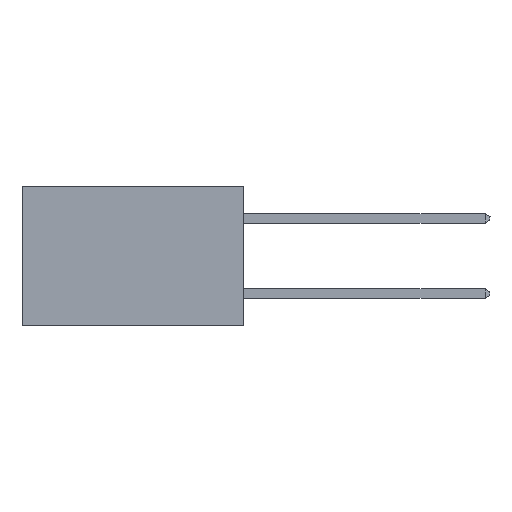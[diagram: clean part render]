
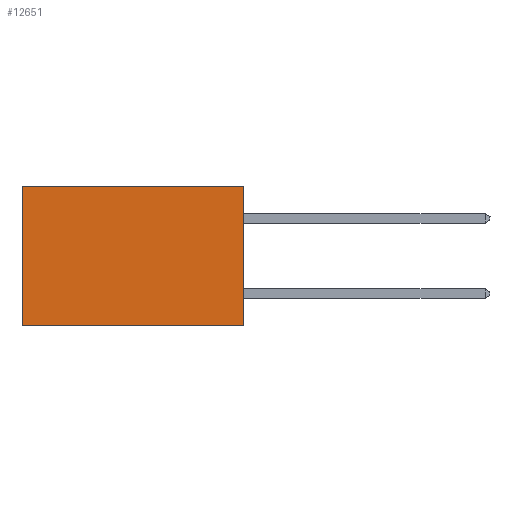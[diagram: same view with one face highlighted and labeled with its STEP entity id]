
A CAD part, left-side view. The second image highlights one B-rep face of the part: STEP entity #12651.
In plain terms, the highlighted planar face has unit normal (-1, 0, 0).
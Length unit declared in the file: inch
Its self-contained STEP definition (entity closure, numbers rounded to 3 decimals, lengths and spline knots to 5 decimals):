
#121 = VERTEX_POINT ( 'NONE', #4408 ) ;
#413 = LINE ( 'NONE', #1261, #7992 ) ;
#588 = CARTESIAN_POINT ( 'NONE',  ( 0.277, 0.59, -0.37 ) ) ;
#641 = CARTESIAN_POINT ( 'NONE',  ( 0.277, 0., -0.37 ) ) ;
#1136 = CARTESIAN_POINT ( 'NONE',  ( 0.277, 0., 0. ) ) ;
#1261 = CARTESIAN_POINT ( 'NONE',  ( 0.277, 0., -0.37 ) ) ;
#1402 = PLANE ( 'NONE',  #4136 ) ;
#2019 = VECTOR ( 'NONE', #10902, 39.37008 ) ;
#2558 = EDGE_CURVE ( 'NONE', #8640, #6250, #5430, .T. ) ;
#2584 = VERTEX_POINT ( 'NONE', #10808 ) ;
#3403 = ORIENTED_EDGE ( 'NONE', *, *, #12127, .T. ) ;
#3412 = DIRECTION ( 'NONE',  ( 1., 0., 0. ) ) ;
#4136 = AXIS2_PLACEMENT_3D ( 'NONE', #9654, #3412, #10673 ) ;
#4408 = CARTESIAN_POINT ( 'NONE',  ( 0.277, 0.59, 0. ) ) ;
#4541 = ORIENTED_EDGE ( 'NONE', *, *, #10246, .T. ) ;
#5396 = CARTESIAN_POINT ( 'NONE',  ( 0.277, 0., -0.37 ) ) ;
#5430 = LINE ( 'NONE', #5396, #8211 ) ;
#5576 = DIRECTION ( 'NONE',  ( 0., 1., 0. ) ) ;
#6250 = VERTEX_POINT ( 'NONE', #641 ) ;
#6359 = ORIENTED_EDGE ( 'NONE', *, *, #10726, .F. ) ;
#6680 = ORIENTED_EDGE ( 'NONE', *, *, #2558, .F. ) ;
#7402 = DIRECTION ( 'NONE',  ( 0., 1., 0. ) ) ;
#7992 = VECTOR ( 'NONE', #7402, 39.37008 ) ;
#8009 = LINE ( 'NONE', #9749, #10441 ) ;
#8211 = VECTOR ( 'NONE', #8912, 39.37008 ) ;
#8640 = VERTEX_POINT ( 'NONE', #1136 ) ;
#8912 = DIRECTION ( 'NONE',  ( 0., 0., -1. ) ) ;
#9593 = FACE_OUTER_BOUND ( 'NONE', #11273, .T. ) ;
#9654 = CARTESIAN_POINT ( 'NONE',  ( 0.277, 0., -0.37 ) ) ;
#9749 = CARTESIAN_POINT ( 'NONE',  ( 0.277, 0., 0. ) ) ;
#10246 = EDGE_CURVE ( 'NONE', #8640, #121, #8009, .T. ) ;
#10251 = LINE ( 'NONE', #588, #2019 ) ;
#10441 = VECTOR ( 'NONE', #5576, 39.37008 ) ;
#10673 = DIRECTION ( 'NONE',  ( 0., 0., -1. ) ) ;
#10726 = EDGE_CURVE ( 'NONE', #6250, #2584, #413, .T. ) ;
#10808 = CARTESIAN_POINT ( 'NONE',  ( 0.277, 0.59, -0.37 ) ) ;
#10902 = DIRECTION ( 'NONE',  ( 0., 0., -1. ) ) ;
#11273 = EDGE_LOOP ( 'NONE', ( #3403, #6359, #6680, #4541 ) ) ;
#12127 = EDGE_CURVE ( 'NONE', #121, #2584, #10251, .T. ) ;
#12651 = ADVANCED_FACE ( 'NONE', ( #9593 ), #1402, .F. ) ;
